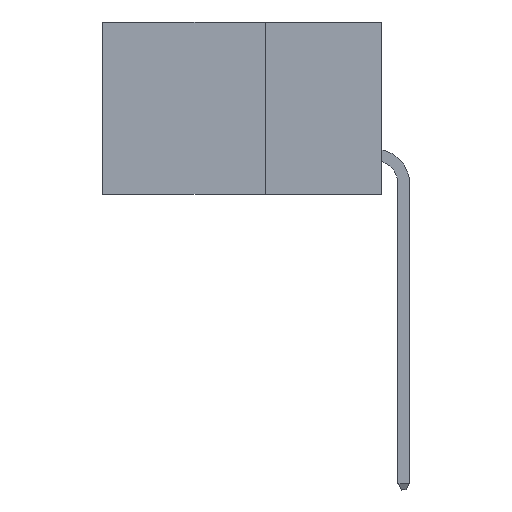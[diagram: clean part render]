
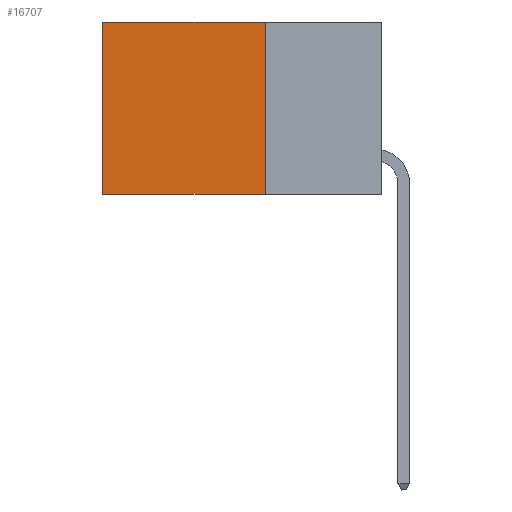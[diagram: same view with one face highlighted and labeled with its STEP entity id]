
A CAD part, left-side view. The second image highlights one B-rep face of the part: STEP entity #16707.
In plain terms, the highlighted planar face has unit normal (-1, 0, 0).
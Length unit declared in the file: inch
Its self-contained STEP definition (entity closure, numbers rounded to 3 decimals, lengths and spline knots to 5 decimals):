
#120 = EDGE_CURVE ( 'NONE', #9168, #14036, #17697, .T. ) ;
#573 = DIRECTION ( 'NONE',  ( 0., 1., 0. ) ) ;
#1150 = LINE ( 'NONE', #7958, #1374 ) ;
#1374 = VECTOR ( 'NONE', #4046, 39.37008 ) ;
#1815 = EDGE_CURVE ( 'NONE', #18484, #14036, #5397, .T. ) ;
#1825 = CARTESIAN_POINT ( 'NONE',  ( 0.2875, 0.25, -0.37 ) ) ;
#2095 = ORIENTED_EDGE ( 'NONE', *, *, #120, .F. ) ;
#2621 = DIRECTION ( 'NONE',  ( 0., 0., -1. ) ) ;
#3259 = DIRECTION ( 'NONE',  ( 0., 1., 0. ) ) ;
#4046 = DIRECTION ( 'NONE',  ( 0., 0., -1. ) ) ;
#4933 = ORIENTED_EDGE ( 'NONE', *, *, #1815, .T. ) ;
#5397 = LINE ( 'NONE', #7470, #17172 ) ;
#7470 = CARTESIAN_POINT ( 'NONE',  ( 0.2875, 0.6, 0. ) ) ;
#7958 = CARTESIAN_POINT ( 'NONE',  ( 0.2875, 0.25, 0. ) ) ;
#8349 = EDGE_CURVE ( 'NONE', #16308, #9168, #1150, .T. ) ;
#8504 = LINE ( 'NONE', #18022, #17596 ) ;
#9168 = VERTEX_POINT ( 'NONE', #16669 ) ;
#10247 = DIRECTION ( 'NONE',  ( 0., 0., -1. ) ) ;
#10389 = CARTESIAN_POINT ( 'NONE',  ( 0.2875, 0.25, 0. ) ) ;
#10654 = CARTESIAN_POINT ( 'NONE',  ( 0.2875, 0.6, -0.37 ) ) ;
#10656 = CARTESIAN_POINT ( 'NONE',  ( 0.2875, 0.6, 0. ) ) ;
#10930 = FACE_OUTER_BOUND ( 'NONE', #15935, .T. ) ;
#12987 = ORIENTED_EDGE ( 'NONE', *, *, #8349, .F. ) ;
#13276 = ORIENTED_EDGE ( 'NONE', *, *, #14655, .T. ) ;
#13777 = VECTOR ( 'NONE', #3259, 39.37008 ) ;
#14036 = VERTEX_POINT ( 'NONE', #10654 ) ;
#14104 = DIRECTION ( 'NONE',  ( 1., 0., 0. ) ) ;
#14633 = AXIS2_PLACEMENT_3D ( 'NONE', #15568, #14104, #2621 ) ;
#14655 = EDGE_CURVE ( 'NONE', #16308, #18484, #8504, .T. ) ;
#15568 = CARTESIAN_POINT ( 'NONE',  ( 0.2875, 0.25, 0. ) ) ;
#15935 = EDGE_LOOP ( 'NONE', ( #4933, #2095, #12987, #13276 ) ) ;
#16308 = VERTEX_POINT ( 'NONE', #10389 ) ;
#16669 = CARTESIAN_POINT ( 'NONE',  ( 0.2875, 0.25, -0.37 ) ) ;
#16707 = ADVANCED_FACE ( 'NONE', ( #10930 ), #16994, .F. ) ;
#16994 = PLANE ( 'NONE',  #14633 ) ;
#17172 = VECTOR ( 'NONE', #10247, 39.37008 ) ;
#17596 = VECTOR ( 'NONE', #573, 39.37008 ) ;
#17697 = LINE ( 'NONE', #1825, #13777 ) ;
#18022 = CARTESIAN_POINT ( 'NONE',  ( 0.2875, 0.25, 0. ) ) ;
#18484 = VERTEX_POINT ( 'NONE', #10656 ) ;
